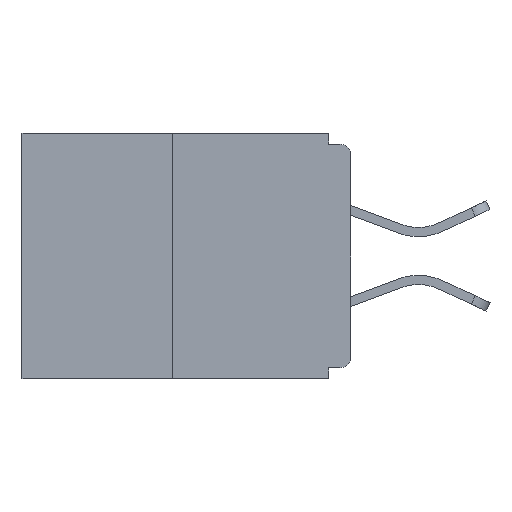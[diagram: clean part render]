
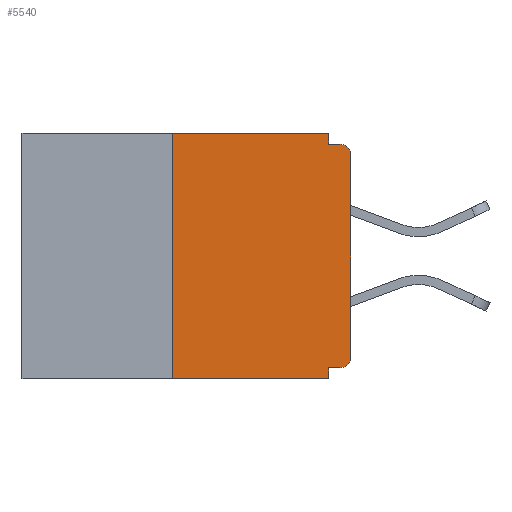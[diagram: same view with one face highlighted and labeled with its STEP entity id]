
A CAD part, left-side view. The second image highlights one B-rep face of the part: STEP entity #5540.
In plain terms, the highlighted planar face has unit normal (-1, 0, 0).
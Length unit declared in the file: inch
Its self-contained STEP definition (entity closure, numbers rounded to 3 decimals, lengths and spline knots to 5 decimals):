
#62 = VECTOR ( 'NONE', #7250, 39.37008 ) ;
#264 = LINE ( 'NONE', #3151, #16997 ) ;
#390 = ORIENTED_EDGE ( 'NONE', *, *, #19384, .T. ) ;
#519 = ORIENTED_EDGE ( 'NONE', *, *, #9669, .F. ) ;
#981 = VECTOR ( 'NONE', #2157, 39.37008 ) ;
#1091 = ORIENTED_EDGE ( 'NONE', *, *, #8202, .F. ) ;
#1318 = EDGE_CURVE ( 'NONE', #11667, #3848, #18511, .T. ) ;
#1773 = VECTOR ( 'NONE', #7538, 39.37008 ) ;
#2062 = VECTOR ( 'NONE', #5180, 39.37008 ) ;
#2157 = DIRECTION ( 'NONE',  ( 0., 0., 1. ) ) ;
#2551 = DIRECTION ( 'NONE',  ( 0., 0., -1. ) ) ;
#2861 = EDGE_CURVE ( 'NONE', #9605, #3848, #9840, .T. ) ;
#2952 = CARTESIAN_POINT ( 'NONE',  ( 0., 0.031, -0.328 ) ) ;
#3151 = CARTESIAN_POINT ( 'NONE',  ( 0., 0.031, -0.343 ) ) ;
#3312 = EDGE_LOOP ( 'NONE', ( #11389, #11300, #16766, #519, #1091, #6713, #390, #14568, #19273, #18669 ) ) ;
#3376 = PLANE ( 'NONE',  #3888 ) ;
#3577 = DIRECTION ( 'NONE',  ( 0., 0., -1. ) ) ;
#3597 = CARTESIAN_POINT ( 'NONE',  ( 0., 0.015, -0.328 ) ) ;
#3729 = FACE_OUTER_BOUND ( 'NONE', #3312, .T. ) ;
#3848 = VERTEX_POINT ( 'NONE', #13239 ) ;
#3888 = AXIS2_PLACEMENT_3D ( 'NONE', #18606, #9607, #3577 ) ;
#4374 = CIRCLE ( 'NONE', #15395, 0.015 ) ;
#5042 = LINE ( 'NONE', #6569, #981 ) ;
#5056 = VECTOR ( 'NONE', #7737, 39.37008 ) ;
#5180 = DIRECTION ( 'NONE',  ( 0., 0., -1. ) ) ;
#5427 = CARTESIAN_POINT ( 'NONE',  ( 0., 0.46, -0.343 ) ) ;
#5489 = CARTESIAN_POINT ( 'NONE',  ( 0., 0., -0.03 ) ) ;
#5540 = ADVANCED_FACE ( 'NONE', ( #3729 ), #3376, .F. ) ;
#5705 = EDGE_CURVE ( 'NONE', #9675, #9605, #12341, .T. ) ;
#6134 = CARTESIAN_POINT ( 'NONE',  ( 0., 0., -0.015 ) ) ;
#6193 = DIRECTION ( 'NONE',  ( 0., -1., 0. ) ) ;
#6569 = CARTESIAN_POINT ( 'NONE',  ( 0., 0.25, 0. ) ) ;
#6713 = ORIENTED_EDGE ( 'NONE', *, *, #18618, .T. ) ;
#7080 = DIRECTION ( 'NONE',  ( -1., 0., 0. ) ) ;
#7250 = DIRECTION ( 'NONE',  ( 0., 0., 1. ) ) ;
#7304 = LINE ( 'NONE', #17090, #9491 ) ;
#7538 = DIRECTION ( 'NONE',  ( 0., 1., 0. ) ) ;
#7737 = DIRECTION ( 'NONE',  ( 0., -1., 0. ) ) ;
#8202 = EDGE_CURVE ( 'NONE', #19034, #10177, #10360, .T. ) ;
#8322 = CARTESIAN_POINT ( 'NONE',  ( 0., 0.031, 0. ) ) ;
#8576 = EDGE_CURVE ( 'NONE', #11876, #19083, #10324, .T. ) ;
#9021 = DIRECTION ( 'NONE',  ( 0., 0., -1. ) ) ;
#9351 = EDGE_CURVE ( 'NONE', #11876, #14742, #5042, .T. ) ;
#9491 = VECTOR ( 'NONE', #6193, 39.37008 ) ;
#9605 = VERTEX_POINT ( 'NONE', #19508 ) ;
#9607 = DIRECTION ( 'NONE',  ( 1., 0., 0. ) ) ;
#9669 = EDGE_CURVE ( 'NONE', #10177, #19083, #264, .T. ) ;
#9675 = VERTEX_POINT ( 'NONE', #18240 ) ;
#9820 = CARTESIAN_POINT ( 'NONE',  ( 0., 0., -0.313 ) ) ;
#9840 = LINE ( 'NONE', #6134, #5056 ) ;
#10113 = CARTESIAN_POINT ( 'NONE',  ( 0., 0., 0. ) ) ;
#10177 = VERTEX_POINT ( 'NONE', #2952 ) ;
#10220 = DIRECTION ( 'NONE',  ( 0., 0., -1. ) ) ;
#10324 = LINE ( 'NONE', #5427, #18937 ) ;
#10360 = LINE ( 'NONE', #15085, #1773 ) ;
#10585 = LINE ( 'NONE', #10113, #62 ) ;
#11300 = ORIENTED_EDGE ( 'NONE', *, *, #9351, .F. ) ;
#11389 = ORIENTED_EDGE ( 'NONE', *, *, #12242, .F. ) ;
#11667 = VERTEX_POINT ( 'NONE', #5489 ) ;
#11864 = AXIS2_PLACEMENT_3D ( 'NONE', #16370, #16306, #2551 ) ;
#11876 = VERTEX_POINT ( 'NONE', #18229 ) ;
#12242 = EDGE_CURVE ( 'NONE', #14742, #9675, #7304, .T. ) ;
#12341 = LINE ( 'NONE', #8322, #2062 ) ;
#12901 = VERTEX_POINT ( 'NONE', #9820 ) ;
#13239 = CARTESIAN_POINT ( 'NONE',  ( 0., 0.015, -0.015 ) ) ;
#14117 = CARTESIAN_POINT ( 'NONE',  ( 0., 0.25, 0. ) ) ;
#14548 = CARTESIAN_POINT ( 'NONE',  ( 0., 0.031, -0.343 ) ) ;
#14568 = ORIENTED_EDGE ( 'NONE', *, *, #1318, .T. ) ;
#14742 = VERTEX_POINT ( 'NONE', #14117 ) ;
#15085 = CARTESIAN_POINT ( 'NONE',  ( 0., 0., -0.328 ) ) ;
#15395 = AXIS2_PLACEMENT_3D ( 'NONE', #19355, #7080, #10220 ) ;
#16306 = DIRECTION ( 'NONE',  ( -1., 0., 0. ) ) ;
#16370 = CARTESIAN_POINT ( 'NONE',  ( 0., 0.015, -0.03 ) ) ;
#16766 = ORIENTED_EDGE ( 'NONE', *, *, #8576, .T. ) ;
#16997 = VECTOR ( 'NONE', #9021, 39.37008 ) ;
#17090 = CARTESIAN_POINT ( 'NONE',  ( 0., 0.46, 0. ) ) ;
#18229 = CARTESIAN_POINT ( 'NONE',  ( 0., 0.25, -0.343 ) ) ;
#18240 = CARTESIAN_POINT ( 'NONE',  ( 0., 0.031, 0. ) ) ;
#18511 = CIRCLE ( 'NONE', #11864, 0.015 ) ;
#18606 = CARTESIAN_POINT ( 'NONE',  ( 0., 0.46, 0. ) ) ;
#18618 = EDGE_CURVE ( 'NONE', #19034, #12901, #4374, .T. ) ;
#18669 = ORIENTED_EDGE ( 'NONE', *, *, #5705, .F. ) ;
#18937 = VECTOR ( 'NONE', #19168, 39.37008 ) ;
#19034 = VERTEX_POINT ( 'NONE', #3597 ) ;
#19083 = VERTEX_POINT ( 'NONE', #14548 ) ;
#19168 = DIRECTION ( 'NONE',  ( 0., -1., 0. ) ) ;
#19273 = ORIENTED_EDGE ( 'NONE', *, *, #2861, .F. ) ;
#19355 = CARTESIAN_POINT ( 'NONE',  ( 0., 0.015, -0.313 ) ) ;
#19384 = EDGE_CURVE ( 'NONE', #12901, #11667, #10585, .T. ) ;
#19508 = CARTESIAN_POINT ( 'NONE',  ( 0., 0.031, -0.015 ) ) ;
